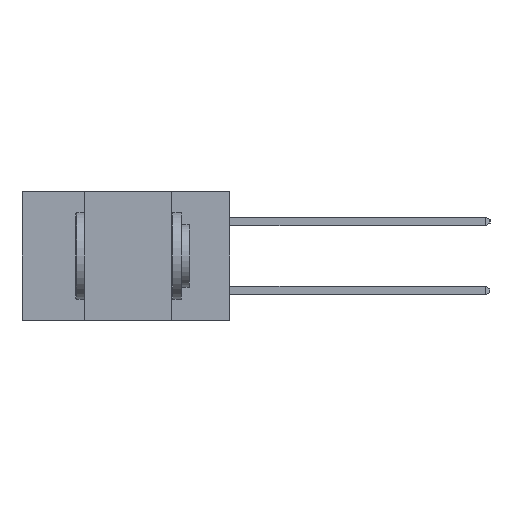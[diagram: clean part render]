
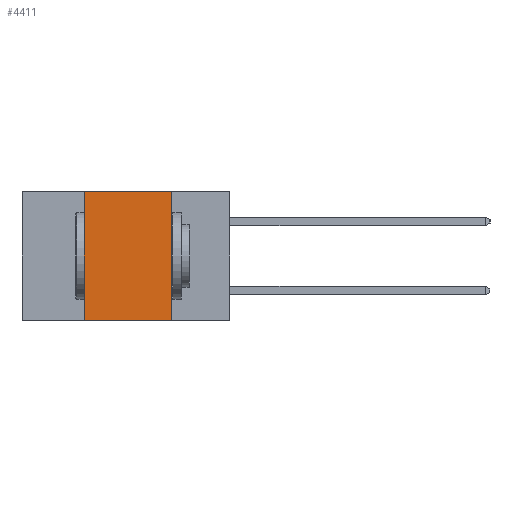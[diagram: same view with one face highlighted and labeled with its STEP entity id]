
A CAD part, left-side view. The second image highlights one B-rep face of the part: STEP entity #4411.
In plain terms, the highlighted planar face has unit normal (-1, 0, 0).
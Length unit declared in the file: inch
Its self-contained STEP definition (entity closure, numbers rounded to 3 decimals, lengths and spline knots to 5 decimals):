
#291 = LINE ( 'NONE', #1246, #11510 ) ;
#1246 = CARTESIAN_POINT ( 'NONE',  ( 0., 0.17, -0.37 ) ) ;
#3729 = ORIENTED_EDGE ( 'NONE', *, *, #7047, .T. ) ;
#4347 = ORIENTED_EDGE ( 'NONE', *, *, #9835, .F. ) ;
#4411 = ADVANCED_FACE ( 'NONE', ( #21136 ), #17954, .F. ) ;
#4773 = CARTESIAN_POINT ( 'NONE',  ( 0., 0.42, 0. ) ) ;
#4989 = CARTESIAN_POINT ( 'NONE',  ( 0., 0.42, -0.37 ) ) ;
#5298 = LINE ( 'NONE', #25894, #11499 ) ;
#7047 = EDGE_CURVE ( 'NONE', #17473, #18190, #18141, .T. ) ;
#7706 = VECTOR ( 'NONE', #25558, 39.37008 ) ;
#8146 = LINE ( 'NONE', #23892, #19900 ) ;
#8874 = CARTESIAN_POINT ( 'NONE',  ( 0., 0.6, -0.37 ) ) ;
#9241 = CARTESIAN_POINT ( 'NONE',  ( 0., 0.17, -0.37 ) ) ;
#9835 = EDGE_CURVE ( 'NONE', #17473, #18090, #5298, .T. ) ;
#10321 = AXIS2_PLACEMENT_3D ( 'NONE', #18290, #17924, #17920 ) ;
#10741 = CARTESIAN_POINT ( 'NONE',  ( 0., 0.17, 0. ) ) ;
#11234 = EDGE_CURVE ( 'NONE', #18090, #21698, #8146, .T. ) ;
#11499 = VECTOR ( 'NONE', #13384, 39.37008 ) ;
#11510 = VECTOR ( 'NONE', #11716, 39.37008 ) ;
#11716 = DIRECTION ( 'NONE',  ( 0., 0., -1. ) ) ;
#12616 = EDGE_CURVE ( 'NONE', #21698, #18190, #291, .T. ) ;
#13384 = DIRECTION ( 'NONE',  ( 0., 0., 1. ) ) ;
#13497 = ORIENTED_EDGE ( 'NONE', *, *, #11234, .F. ) ;
#17473 = VERTEX_POINT ( 'NONE', #4989 ) ;
#17920 = DIRECTION ( 'NONE',  ( 0., 0., -1. ) ) ;
#17924 = DIRECTION ( 'NONE',  ( 1., 0., 0. ) ) ;
#17954 = PLANE ( 'NONE',  #10321 ) ;
#18090 = VERTEX_POINT ( 'NONE', #4773 ) ;
#18141 = LINE ( 'NONE', #8874, #7706 ) ;
#18190 = VERTEX_POINT ( 'NONE', #9241 ) ;
#18290 = CARTESIAN_POINT ( 'NONE',  ( 0., 0.6, 0. ) ) ;
#19900 = VECTOR ( 'NONE', #25996, 39.37008 ) ;
#21136 = FACE_OUTER_BOUND ( 'NONE', #25014, .T. ) ;
#21698 = VERTEX_POINT ( 'NONE', #10741 ) ;
#23892 = CARTESIAN_POINT ( 'NONE',  ( 0., 0.6, 0. ) ) ;
#25014 = EDGE_LOOP ( 'NONE', ( #25719, #13497, #4347, #3729 ) ) ;
#25558 = DIRECTION ( 'NONE',  ( 0., -1., 0. ) ) ;
#25719 = ORIENTED_EDGE ( 'NONE', *, *, #12616, .F. ) ;
#25894 = CARTESIAN_POINT ( 'NONE',  ( 0., 0.42, -0.37 ) ) ;
#25996 = DIRECTION ( 'NONE',  ( 0., -1., 0. ) ) ;
